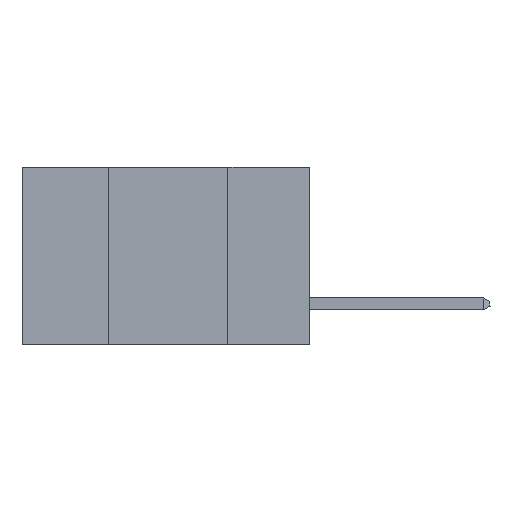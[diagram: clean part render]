
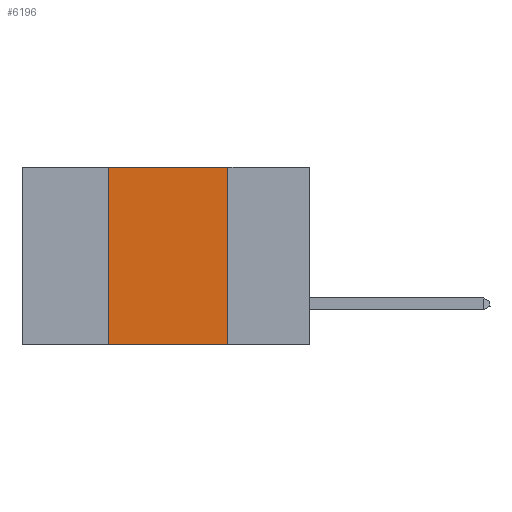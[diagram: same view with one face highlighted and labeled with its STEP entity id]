
A CAD part, left-side view. The second image highlights one B-rep face of the part: STEP entity #6196.
In plain terms, the highlighted planar face has unit normal (-1, 0, 0).
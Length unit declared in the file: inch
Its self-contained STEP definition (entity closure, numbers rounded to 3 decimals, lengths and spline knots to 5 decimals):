
#20 = DIRECTION ( 'NONE',  ( 1., 0., 0. ) ) ;
#88 = CARTESIAN_POINT ( 'NONE',  ( 0., 0.17, -0.37 ) ) ;
#127 = CARTESIAN_POINT ( 'NONE',  ( 0., 0.42, 0. ) ) ;
#167 = EDGE_CURVE ( 'NONE', #2663, #10331, #17214, .T. ) ;
#2525 = FACE_OUTER_BOUND ( 'NONE', #15894, .T. ) ;
#2663 = VERTEX_POINT ( 'NONE', #127 ) ;
#3069 = EDGE_CURVE ( 'NONE', #10331, #18771, #4715, .T. ) ;
#3267 = CARTESIAN_POINT ( 'NONE',  ( 0., 0.6, 0. ) ) ;
#3294 = CARTESIAN_POINT ( 'NONE',  ( 0., 0.42, -0.37 ) ) ;
#4475 = VERTEX_POINT ( 'NONE', #3294 ) ;
#4699 = PLANE ( 'NONE',  #14285 ) ;
#4715 = LINE ( 'NONE', #11896, #11565 ) ;
#5058 = LINE ( 'NONE', #15566, #17988 ) ;
#6196 = ADVANCED_FACE ( 'NONE', ( #2525 ), #4699, .F. ) ;
#6413 = VECTOR ( 'NONE', #7435, 39.37008 ) ;
#7240 = CARTESIAN_POINT ( 'NONE',  ( 0., 0.17, 0. ) ) ;
#7435 = DIRECTION ( 'NONE',  ( 0., 0., 1. ) ) ;
#7631 = ORIENTED_EDGE ( 'NONE', *, *, #3069, .F. ) ;
#10286 = EDGE_CURVE ( 'NONE', #4475, #2663, #15844, .T. ) ;
#10331 = VERTEX_POINT ( 'NONE', #7240 ) ;
#11565 = VECTOR ( 'NONE', #16378, 39.37008 ) ;
#11896 = CARTESIAN_POINT ( 'NONE',  ( 0., 0.17, 0. ) ) ;
#12517 = VECTOR ( 'NONE', #12693, 39.37008 ) ;
#12693 = DIRECTION ( 'NONE',  ( 0., -1., 0. ) ) ;
#12836 = CARTESIAN_POINT ( 'NONE',  ( 0., 0.6, 0. ) ) ;
#14285 = AXIS2_PLACEMENT_3D ( 'NONE', #3267, #20, #16472 ) ;
#15566 = CARTESIAN_POINT ( 'NONE',  ( 0., 0.6, -0.37 ) ) ;
#15844 = LINE ( 'NONE', #16440, #6413 ) ;
#15894 = EDGE_LOOP ( 'NONE', ( #7631, #18723, #16722, #18621 ) ) ;
#16378 = DIRECTION ( 'NONE',  ( 0., 0., -1. ) ) ;
#16440 = CARTESIAN_POINT ( 'NONE',  ( 0., 0.42, 0. ) ) ;
#16472 = DIRECTION ( 'NONE',  ( 0., 0., -1. ) ) ;
#16592 = EDGE_CURVE ( 'NONE', #4475, #18771, #5058, .T. ) ;
#16722 = ORIENTED_EDGE ( 'NONE', *, *, #10286, .F. ) ;
#17130 = DIRECTION ( 'NONE',  ( 0., -1., 0. ) ) ;
#17214 = LINE ( 'NONE', #12836, #12517 ) ;
#17988 = VECTOR ( 'NONE', #17130, 39.37008 ) ;
#18621 = ORIENTED_EDGE ( 'NONE', *, *, #16592, .T. ) ;
#18723 = ORIENTED_EDGE ( 'NONE', *, *, #167, .F. ) ;
#18771 = VERTEX_POINT ( 'NONE', #88 ) ;
